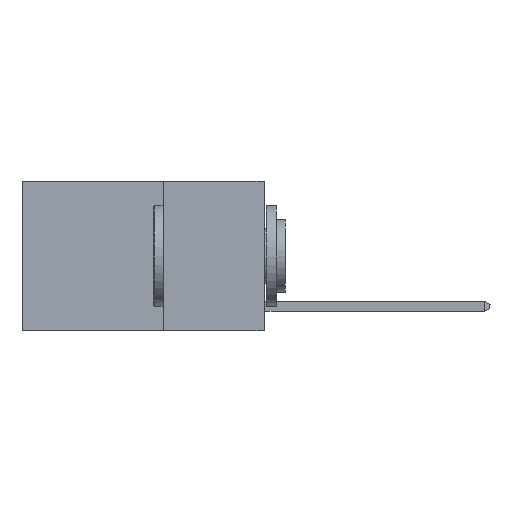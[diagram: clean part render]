
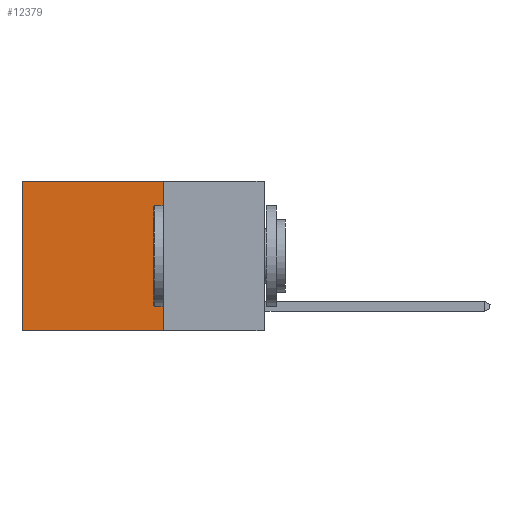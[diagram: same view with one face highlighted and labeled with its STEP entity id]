
A CAD part, left-side view. The second image highlights one B-rep face of the part: STEP entity #12379.
In plain terms, the highlighted planar face has unit normal (-1, 0, 0).
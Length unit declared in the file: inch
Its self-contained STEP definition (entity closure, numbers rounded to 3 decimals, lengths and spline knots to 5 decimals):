
#140 = VECTOR ( 'NONE', #794, 39.37008 ) ;
#794 = DIRECTION ( 'NONE',  ( 0., 0., -1. ) ) ;
#1087 = CARTESIAN_POINT ( 'NONE',  ( 0.2625, 0.25, 0. ) ) ;
#1316 = DIRECTION ( 'NONE',  ( 0., 0., -1. ) ) ;
#2474 = DIRECTION ( 'NONE',  ( 0., 0., -1. ) ) ;
#2783 = DIRECTION ( 'NONE',  ( 0., 1., 0. ) ) ;
#3597 = VERTEX_POINT ( 'NONE', #9206 ) ;
#4284 = LINE ( 'NONE', #15031, #4474 ) ;
#4474 = VECTOR ( 'NONE', #19688, 39.37008 ) ;
#5214 = AXIS2_PLACEMENT_3D ( 'NONE', #10690, #16815, #1316 ) ;
#5685 = ORIENTED_EDGE ( 'NONE', *, *, #14099, .F. ) ;
#5801 = VERTEX_POINT ( 'NONE', #15695 ) ;
#6147 = VERTEX_POINT ( 'NONE', #11147 ) ;
#6398 = CARTESIAN_POINT ( 'NONE',  ( 0.2625, 0.6, -0.37 ) ) ;
#7123 = CARTESIAN_POINT ( 'NONE',  ( 0.2625, 0.6, 0. ) ) ;
#7525 = ORIENTED_EDGE ( 'NONE', *, *, #9213, .F. ) ;
#8770 = LINE ( 'NONE', #1087, #140 ) ;
#9009 = VECTOR ( 'NONE', #2474, 39.37008 ) ;
#9206 = CARTESIAN_POINT ( 'NONE',  ( 0.2625, 0.6, 0. ) ) ;
#9213 = EDGE_CURVE ( 'NONE', #6147, #17713, #4284, .T. ) ;
#10276 = EDGE_CURVE ( 'NONE', #3597, #17713, #11756, .T. ) ;
#10690 = CARTESIAN_POINT ( 'NONE',  ( 0.2625, 0.25, 0. ) ) ;
#11147 = CARTESIAN_POINT ( 'NONE',  ( 0.2625, 0.25, -0.37 ) ) ;
#11756 = LINE ( 'NONE', #7123, #9009 ) ;
#12379 = ADVANCED_FACE ( 'NONE', ( #13594 ), #13680, .F. ) ;
#13594 = FACE_OUTER_BOUND ( 'NONE', #14822, .T. ) ;
#13680 = PLANE ( 'NONE',  #5214 ) ;
#13771 = VECTOR ( 'NONE', #2783, 39.37008 ) ;
#14099 = EDGE_CURVE ( 'NONE', #5801, #6147, #8770, .T. ) ;
#14366 = ORIENTED_EDGE ( 'NONE', *, *, #18778, .T. ) ;
#14822 = EDGE_LOOP ( 'NONE', ( #16696, #7525, #5685, #14366 ) ) ;
#15031 = CARTESIAN_POINT ( 'NONE',  ( 0.2625, 0.25, -0.37 ) ) ;
#15251 = LINE ( 'NONE', #16572, #13771 ) ;
#15695 = CARTESIAN_POINT ( 'NONE',  ( 0.2625, 0.25, 0. ) ) ;
#16572 = CARTESIAN_POINT ( 'NONE',  ( 0.2625, 0.25, 0. ) ) ;
#16696 = ORIENTED_EDGE ( 'NONE', *, *, #10276, .T. ) ;
#16815 = DIRECTION ( 'NONE',  ( 1., 0., 0. ) ) ;
#17713 = VERTEX_POINT ( 'NONE', #6398 ) ;
#18778 = EDGE_CURVE ( 'NONE', #5801, #3597, #15251, .T. ) ;
#19688 = DIRECTION ( 'NONE',  ( 0., 1., 0. ) ) ;
